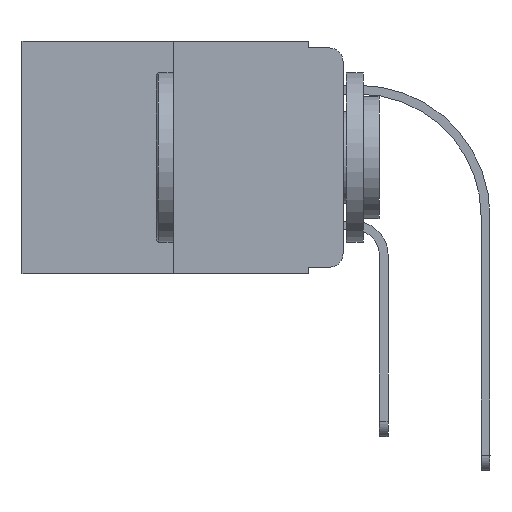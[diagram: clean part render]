
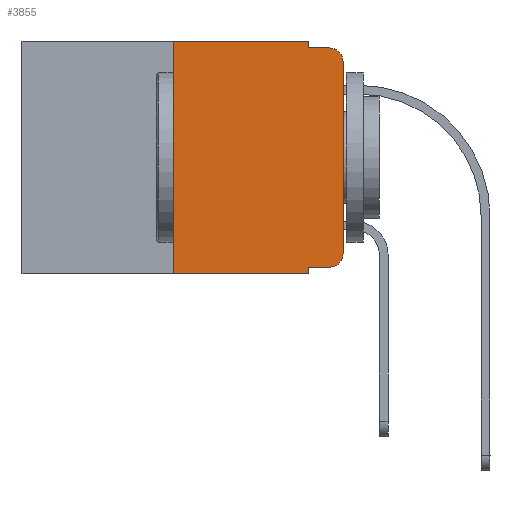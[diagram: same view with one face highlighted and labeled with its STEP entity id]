
A CAD part, left-side view. The second image highlights one B-rep face of the part: STEP entity #3855.
In plain terms, the highlighted planar face has unit normal (-1, 0, 0).
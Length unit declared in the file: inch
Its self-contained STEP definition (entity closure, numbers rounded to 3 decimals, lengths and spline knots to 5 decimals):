
#1027 = CARTESIAN_POINT ( 'NONE',  ( 0., 0.02, -0.01 ) ) ;
#1126 = DIRECTION ( 'NONE',  ( 0., -1., 0. ) ) ;
#1147 = VERTEX_POINT ( 'NONE', #2970 ) ;
#1361 = ORIENTED_EDGE ( 'NONE', *, *, #13682, .F. ) ;
#1448 = VECTOR ( 'NONE', #4413, 39.37008 ) ;
#1497 = DIRECTION ( 'NONE',  ( 0., 0., 1. ) ) ;
#1657 = LINE ( 'NONE', #7420, #4846 ) ;
#1748 = DIRECTION ( 'NONE',  ( 0., 0., -1. ) ) ;
#1840 = DIRECTION ( 'NONE',  ( 0., -1., 0. ) ) ;
#2384 = CARTESIAN_POINT ( 'NONE',  ( 0., 0.051, -0.333 ) ) ;
#2527 = CIRCLE ( 'NONE', #9078, 0.02 ) ;
#2970 = CARTESIAN_POINT ( 'NONE',  ( 0., 0.25, 0. ) ) ;
#3094 = PLANE ( 'NONE',  #12065 ) ;
#3159 = CARTESIAN_POINT ( 'NONE',  ( 0., 0., -0.313 ) ) ;
#3522 = ORIENTED_EDGE ( 'NONE', *, *, #11395, .T. ) ;
#3573 = LINE ( 'NONE', #7866, #8437 ) ;
#3720 = ORIENTED_EDGE ( 'NONE', *, *, #11596, .T. ) ;
#3855 = ADVANCED_FACE ( 'NONE', ( #5687 ), #3094, .F. ) ;
#3955 = VECTOR ( 'NONE', #1126, 39.37008 ) ;
#4050 = CARTESIAN_POINT ( 'NONE',  ( 0., 0.25, 0. ) ) ;
#4413 = DIRECTION ( 'NONE',  ( 0., 0., 1. ) ) ;
#4808 = EDGE_LOOP ( 'NONE', ( #3720, #7644, #5019, #5343, #15708, #7009, #9978, #1361, #8311, #3522 ) ) ;
#4846 = VECTOR ( 'NONE', #1748, 39.37008 ) ;
#4874 = EDGE_CURVE ( 'NONE', #17622, #13811, #1657, .T. ) ;
#4975 = CARTESIAN_POINT ( 'NONE',  ( 0., 0.25, -0.343 ) ) ;
#5019 = ORIENTED_EDGE ( 'NONE', *, *, #16907, .F. ) ;
#5090 = LINE ( 'NONE', #10787, #17756 ) ;
#5183 = DIRECTION ( 'NONE',  ( 0., 0., -1. ) ) ;
#5343 = ORIENTED_EDGE ( 'NONE', *, *, #4874, .F. ) ;
#5384 = CARTESIAN_POINT ( 'NONE',  ( 0., 0.473, -0.343 ) ) ;
#5424 = VERTEX_POINT ( 'NONE', #10557 ) ;
#5687 = FACE_OUTER_BOUND ( 'NONE', #4808, .T. ) ;
#6081 = DIRECTION ( 'NONE',  ( 0., 0., -1. ) ) ;
#6180 = VERTEX_POINT ( 'NONE', #11730 ) ;
#6835 = VERTEX_POINT ( 'NONE', #4975 ) ;
#6839 = EDGE_CURVE ( 'NONE', #1147, #17622, #3573, .T. ) ;
#7009 = ORIENTED_EDGE ( 'NONE', *, *, #10273, .F. ) ;
#7217 = CARTESIAN_POINT ( 'NONE',  ( 0., 0.051, -0.01 ) ) ;
#7420 = CARTESIAN_POINT ( 'NONE',  ( 0., 0.051, 0. ) ) ;
#7644 = ORIENTED_EDGE ( 'NONE', *, *, #12694, .T. ) ;
#7866 = CARTESIAN_POINT ( 'NONE',  ( 0., 0.473, 0. ) ) ;
#7891 = DIRECTION ( 'NONE',  ( 0., 0., -1. ) ) ;
#8185 = VERTEX_POINT ( 'NONE', #3159 ) ;
#8311 = ORIENTED_EDGE ( 'NONE', *, *, #10076, .T. ) ;
#8369 = LINE ( 'NONE', #13128, #17311 ) ;
#8437 = VECTOR ( 'NONE', #13572, 39.37008 ) ;
#9078 = AXIS2_PLACEMENT_3D ( 'NONE', #17836, #14663, #6081 ) ;
#9621 = VERTEX_POINT ( 'NONE', #17809 ) ;
#9978 = ORIENTED_EDGE ( 'NONE', *, *, #18011, .T. ) ;
#10076 = EDGE_CURVE ( 'NONE', #9621, #5424, #15171, .T. ) ;
#10273 = EDGE_CURVE ( 'NONE', #6835, #1147, #15357, .T. ) ;
#10557 = CARTESIAN_POINT ( 'NONE',  ( 0., 0.02, -0.333 ) ) ;
#10725 = LINE ( 'NONE', #5384, #3955 ) ;
#10768 = CARTESIAN_POINT ( 'NONE',  ( 0., 0.051, 0. ) ) ;
#10787 = CARTESIAN_POINT ( 'NONE',  ( 0., 0.051, 0. ) ) ;
#10887 = DIRECTION ( 'NONE',  ( -1., 0., 0. ) ) ;
#11395 = EDGE_CURVE ( 'NONE', #5424, #8185, #15109, .T. ) ;
#11596 = EDGE_CURVE ( 'NONE', #8185, #6180, #14362, .T. ) ;
#11730 = CARTESIAN_POINT ( 'NONE',  ( 0., 0., -0.03 ) ) ;
#12065 = AXIS2_PLACEMENT_3D ( 'NONE', #15881, #15700, #14385 ) ;
#12694 = EDGE_CURVE ( 'NONE', #6180, #13341, #2527, .T. ) ;
#13087 = VERTEX_POINT ( 'NONE', #17628 ) ;
#13128 = CARTESIAN_POINT ( 'NONE',  ( 0., 0.051, -0.01 ) ) ;
#13341 = VERTEX_POINT ( 'NONE', #1027 ) ;
#13572 = DIRECTION ( 'NONE',  ( 0., -1., 0. ) ) ;
#13682 = EDGE_CURVE ( 'NONE', #9621, #13087, #5090, .T. ) ;
#13811 = VERTEX_POINT ( 'NONE', #7217 ) ;
#14187 = CARTESIAN_POINT ( 'NONE',  ( 0., 0., 0. ) ) ;
#14209 = AXIS2_PLACEMENT_3D ( 'NONE', #18068, #10887, #7891 ) ;
#14362 = LINE ( 'NONE', #14187, #15902 ) ;
#14385 = DIRECTION ( 'NONE',  ( 0., 0., -1. ) ) ;
#14663 = DIRECTION ( 'NONE',  ( -1., 0., 0. ) ) ;
#14804 = DIRECTION ( 'NONE',  ( 0., -1., 0. ) ) ;
#15109 = CIRCLE ( 'NONE', #14209, 0.02 ) ;
#15171 = LINE ( 'NONE', #2384, #16349 ) ;
#15357 = LINE ( 'NONE', #4050, #1448 ) ;
#15700 = DIRECTION ( 'NONE',  ( 1., 0., 0. ) ) ;
#15708 = ORIENTED_EDGE ( 'NONE', *, *, #6839, .F. ) ;
#15881 = CARTESIAN_POINT ( 'NONE',  ( 0., 0.473, 0. ) ) ;
#15902 = VECTOR ( 'NONE', #1497, 39.37008 ) ;
#16349 = VECTOR ( 'NONE', #14804, 39.37008 ) ;
#16907 = EDGE_CURVE ( 'NONE', #13811, #13341, #8369, .T. ) ;
#17311 = VECTOR ( 'NONE', #1840, 39.37008 ) ;
#17622 = VERTEX_POINT ( 'NONE', #10768 ) ;
#17628 = CARTESIAN_POINT ( 'NONE',  ( 0., 0.051, -0.343 ) ) ;
#17756 = VECTOR ( 'NONE', #5183, 39.37008 ) ;
#17809 = CARTESIAN_POINT ( 'NONE',  ( 0., 0.051, -0.333 ) ) ;
#17836 = CARTESIAN_POINT ( 'NONE',  ( 0., 0.02, -0.03 ) ) ;
#18011 = EDGE_CURVE ( 'NONE', #6835, #13087, #10725, .T. ) ;
#18068 = CARTESIAN_POINT ( 'NONE',  ( 0., 0.02, -0.313 ) ) ;
